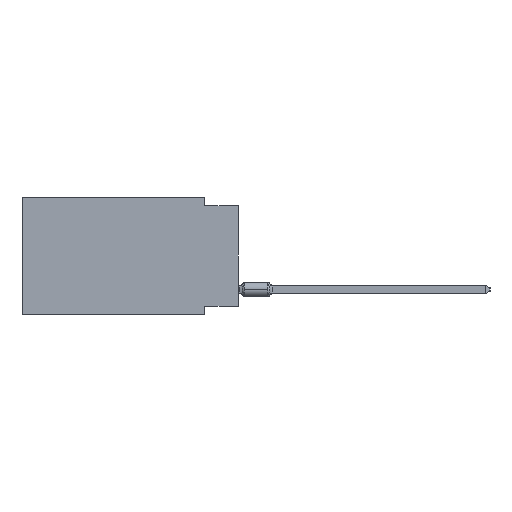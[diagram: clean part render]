
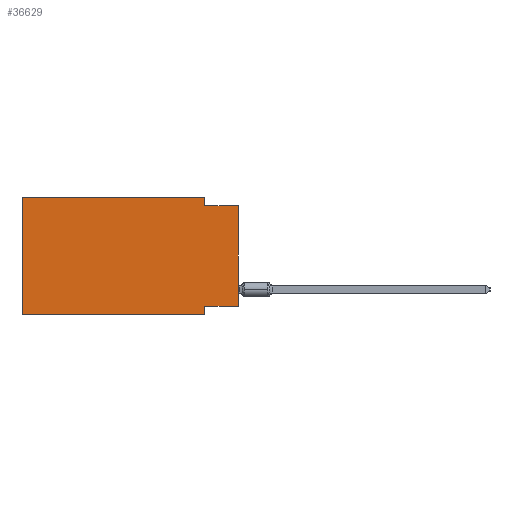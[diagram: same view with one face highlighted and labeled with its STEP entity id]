
A CAD part, left-side view. The second image highlights one B-rep face of the part: STEP entity #36629.
In plain terms, the highlighted planar face has unit normal (-1, 0, 0).
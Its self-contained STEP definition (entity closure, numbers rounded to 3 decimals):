
#765 = PLANE ( 'NONE',  #26821 ) ;
#1143 = VECTOR ( 'NONE', #96504, 1000. ) ;
#1317 = CARTESIAN_POINT ( 'NONE',  ( 0., 16.383, 0. ) ) ;
#1330 = EDGE_CURVE ( 'NONE', #29608, #91565, #61530, .T. ) ;
#2793 = VERTEX_POINT ( 'NONE', #93005 ) ;
#3418 = VECTOR ( 'NONE', #80793, 1000. ) ;
#3444 = CARTESIAN_POINT ( 'NONE',  ( 0., 16.383, 0. ) ) ;
#5174 = CARTESIAN_POINT ( 'NONE',  ( 0., 16.383, -8.89 ) ) ;
#5473 = EDGE_CURVE ( 'NONE', #9839, #13518, #51108, .T. ) ;
#8651 = EDGE_CURVE ( 'NONE', #29608, #61564, #57282, .T. ) ;
#9839 = VERTEX_POINT ( 'NONE', #95805 ) ;
#11808 = ORIENTED_EDGE ( 'NONE', *, *, #40426, .F. ) ;
#13518 = VERTEX_POINT ( 'NONE', #35732 ) ;
#13701 = LINE ( 'NONE', #91608, #80143 ) ;
#15665 = ORIENTED_EDGE ( 'NONE', *, *, #106299, .T. ) ;
#16242 = VECTOR ( 'NONE', #93525, 1000. ) ;
#16555 = LINE ( 'NONE', #17135, #61678 ) ;
#17135 = CARTESIAN_POINT ( 'NONE',  ( 0., 2.54, -8.89 ) ) ;
#17607 = EDGE_CURVE ( 'NONE', #13518, #28979, #31053, .T. ) ;
#21142 = DIRECTION ( 'NONE',  ( 0., 1., 0. ) ) ;
#25889 = VECTOR ( 'NONE', #100950, 1000. ) ;
#26821 = AXIS2_PLACEMENT_3D ( 'NONE', #1317, #69488, #60899 ) ;
#28979 = VERTEX_POINT ( 'NONE', #104732 ) ;
#29608 = VERTEX_POINT ( 'NONE', #92486 ) ;
#31053 = LINE ( 'NONE', #65984, #25889 ) ;
#32779 = CARTESIAN_POINT ( 'NONE',  ( 0., 2.54, 0. ) ) ;
#35732 = CARTESIAN_POINT ( 'NONE',  ( 0., 2.54, -0.635 ) ) ;
#36276 = ORIENTED_EDGE ( 'NONE', *, *, #8651, .T. ) ;
#36629 = ADVANCED_FACE ( 'NONE', ( #60326 ), #765, .F. ) ;
#38852 = VECTOR ( 'NONE', #98150, 1000. ) ;
#40426 = EDGE_CURVE ( 'NONE', #2793, #72991, #13701, .T. ) ;
#42729 = VECTOR ( 'NONE', #93367, 1000. ) ;
#44349 = CARTESIAN_POINT ( 'NONE',  ( 0., 0., 0. ) ) ;
#46801 = CARTESIAN_POINT ( 'NONE',  ( 0., 16.383, 0. ) ) ;
#51108 = LINE ( 'NONE', #32779, #16242 ) ;
#52926 = LINE ( 'NONE', #44349, #38852 ) ;
#57282 = LINE ( 'NONE', #5174, #42729 ) ;
#58838 = ORIENTED_EDGE ( 'NONE', *, *, #79143, .F. ) ;
#60326 = FACE_OUTER_BOUND ( 'NONE', #72437, .T. ) ;
#60899 = DIRECTION ( 'NONE',  ( 0., 0., -1. ) ) ;
#61530 = LINE ( 'NONE', #86233, #1143 ) ;
#61564 = VERTEX_POINT ( 'NONE', #92898 ) ;
#61678 = VECTOR ( 'NONE', #96752, 1000. ) ;
#65675 = ORIENTED_EDGE ( 'NONE', *, *, #5473, .F. ) ;
#65984 = CARTESIAN_POINT ( 'NONE',  ( 0., 0., -0.635 ) ) ;
#67246 = ORIENTED_EDGE ( 'NONE', *, *, #1330, .F. ) ;
#69488 = DIRECTION ( 'NONE',  ( 1., 0., 0. ) ) ;
#72437 = EDGE_LOOP ( 'NONE', ( #15665, #99914, #65675, #78164, #67246, #36276, #58838, #11808 ) ) ;
#72991 = VERTEX_POINT ( 'NONE', #112578 ) ;
#78164 = ORIENTED_EDGE ( 'NONE', *, *, #92223, .F. ) ;
#79143 = EDGE_CURVE ( 'NONE', #72991, #61564, #16555, .T. ) ;
#80143 = VECTOR ( 'NONE', #21142, 1000. ) ;
#80793 = DIRECTION ( 'NONE',  ( 0., -1., 0. ) ) ;
#86233 = CARTESIAN_POINT ( 'NONE',  ( 0., 16.383, 0. ) ) ;
#91565 = VERTEX_POINT ( 'NONE', #46801 ) ;
#91608 = CARTESIAN_POINT ( 'NONE',  ( 0., 0., -8.255 ) ) ;
#92223 = EDGE_CURVE ( 'NONE', #91565, #9839, #98530, .T. ) ;
#92486 = CARTESIAN_POINT ( 'NONE',  ( 0., 16.383, -8.89 ) ) ;
#92898 = CARTESIAN_POINT ( 'NONE',  ( 0., 2.54, -8.89 ) ) ;
#93005 = CARTESIAN_POINT ( 'NONE',  ( 0., 0., -8.255 ) ) ;
#93367 = DIRECTION ( 'NONE',  ( 0., -1., 0. ) ) ;
#93525 = DIRECTION ( 'NONE',  ( 0., 0., -1. ) ) ;
#95805 = CARTESIAN_POINT ( 'NONE',  ( 0., 2.54, 0. ) ) ;
#96504 = DIRECTION ( 'NONE',  ( 0., 0., 1. ) ) ;
#96752 = DIRECTION ( 'NONE',  ( 0., 0., -1. ) ) ;
#98150 = DIRECTION ( 'NONE',  ( 0., 0., 1. ) ) ;
#98530 = LINE ( 'NONE', #3444, #3418 ) ;
#99914 = ORIENTED_EDGE ( 'NONE', *, *, #17607, .F. ) ;
#100950 = DIRECTION ( 'NONE',  ( 0., -1., 0. ) ) ;
#104732 = CARTESIAN_POINT ( 'NONE',  ( 0., 0., -0.635 ) ) ;
#106299 = EDGE_CURVE ( 'NONE', #2793, #28979, #52926, .T. ) ;
#112578 = CARTESIAN_POINT ( 'NONE',  ( 0., 2.54, -8.255 ) ) ;
